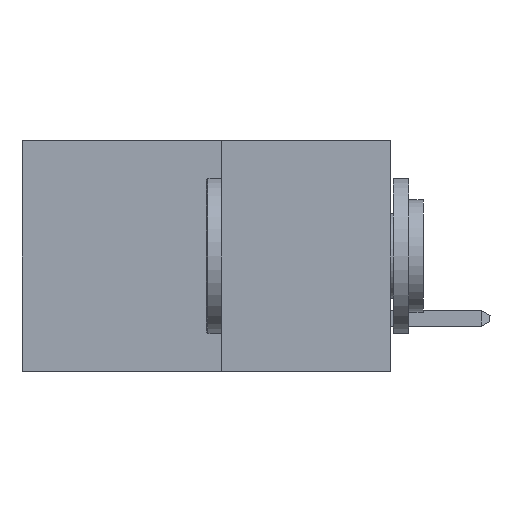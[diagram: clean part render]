
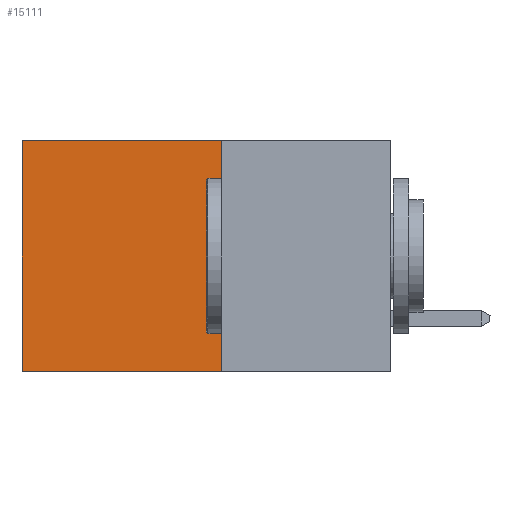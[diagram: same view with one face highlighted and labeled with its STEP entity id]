
A CAD part, left-side view. The second image highlights one B-rep face of the part: STEP entity #15111.
In plain terms, the highlighted planar face has unit normal (-1, 0, 0).
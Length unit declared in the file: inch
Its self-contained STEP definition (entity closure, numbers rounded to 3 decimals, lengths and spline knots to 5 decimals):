
#251 = ORIENTED_EDGE ( 'NONE', *, *, #4827, .F. ) ;
#865 = ORIENTED_EDGE ( 'NONE', *, *, #15337, .F. ) ;
#1435 = CARTESIAN_POINT ( 'NONE',  ( 0.277, 0.59, -0.37 ) ) ;
#1731 = DIRECTION ( 'NONE',  ( 0., 0., -1. ) ) ;
#1803 = CARTESIAN_POINT ( 'NONE',  ( 0.277, 0.27, -0.37 ) ) ;
#2827 = CARTESIAN_POINT ( 'NONE',  ( 0.277, 0.59, 0. ) ) ;
#2908 = VERTEX_POINT ( 'NONE', #12391 ) ;
#3164 = LINE ( 'NONE', #1435, #19723 ) ;
#3181 = CARTESIAN_POINT ( 'NONE',  ( 0.277, 0.27, 0. ) ) ;
#4016 = LINE ( 'NONE', #8955, #13548 ) ;
#4822 = EDGE_LOOP ( 'NONE', ( #10705, #251, #865, #18931 ) ) ;
#4827 = EDGE_CURVE ( 'NONE', #2908, #9354, #4016, .T. ) ;
#4879 = DIRECTION ( 'NONE',  ( 0., 1., 0. ) ) ;
#5881 = AXIS2_PLACEMENT_3D ( 'NONE', #17875, #8067, #19473 ) ;
#6307 = PLANE ( 'NONE',  #5881 ) ;
#7143 = VECTOR ( 'NONE', #1731, 39.37008 ) ;
#7673 = LINE ( 'NONE', #3181, #16436 ) ;
#8067 = DIRECTION ( 'NONE',  ( 1., 0., 0. ) ) ;
#8955 = CARTESIAN_POINT ( 'NONE',  ( 0.277, 0.27, -0.37 ) ) ;
#8995 = DIRECTION ( 'NONE',  ( 0., 1., 0. ) ) ;
#9354 = VERTEX_POINT ( 'NONE', #10400 ) ;
#10400 = CARTESIAN_POINT ( 'NONE',  ( 0.277, 0.59, -0.37 ) ) ;
#10705 = ORIENTED_EDGE ( 'NONE', *, *, #11619, .T. ) ;
#11526 = CARTESIAN_POINT ( 'NONE',  ( 0.277, 0.27, 0. ) ) ;
#11619 = EDGE_CURVE ( 'NONE', #12155, #9354, #3164, .T. ) ;
#11671 = DIRECTION ( 'NONE',  ( 0., 0., -1. ) ) ;
#12155 = VERTEX_POINT ( 'NONE', #2827 ) ;
#12391 = CARTESIAN_POINT ( 'NONE',  ( 0.277, 0.27, -0.37 ) ) ;
#12850 = EDGE_CURVE ( 'NONE', #13986, #12155, #7673, .T. ) ;
#13548 = VECTOR ( 'NONE', #8995, 39.37008 ) ;
#13986 = VERTEX_POINT ( 'NONE', #11526 ) ;
#15111 = ADVANCED_FACE ( 'NONE', ( #20637 ), #6307, .F. ) ;
#15337 = EDGE_CURVE ( 'NONE', #13986, #2908, #15950, .T. ) ;
#15950 = LINE ( 'NONE', #1803, #7143 ) ;
#16436 = VECTOR ( 'NONE', #4879, 39.37008 ) ;
#17875 = CARTESIAN_POINT ( 'NONE',  ( 0.277, 0.27, -0.37 ) ) ;
#18931 = ORIENTED_EDGE ( 'NONE', *, *, #12850, .T. ) ;
#19473 = DIRECTION ( 'NONE',  ( 0., 0., -1. ) ) ;
#19723 = VECTOR ( 'NONE', #11671, 39.37008 ) ;
#20637 = FACE_OUTER_BOUND ( 'NONE', #4822, .T. ) ;
